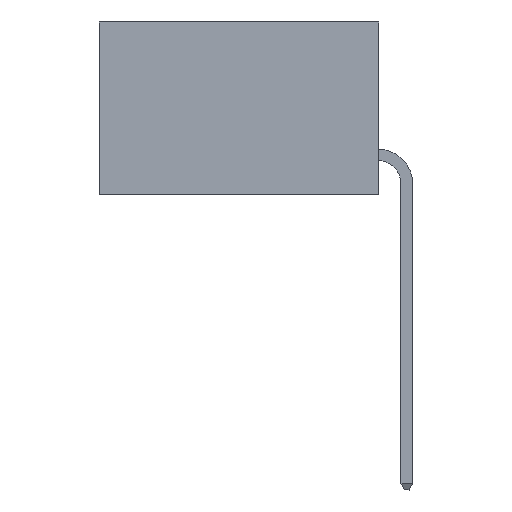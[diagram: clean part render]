
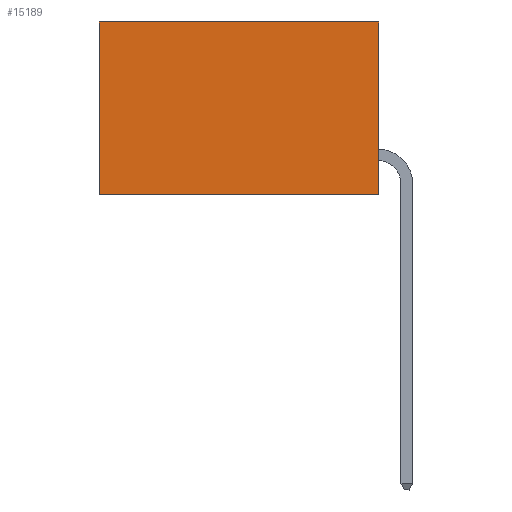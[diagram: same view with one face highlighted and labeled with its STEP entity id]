
A CAD part, left-side view. The second image highlights one B-rep face of the part: STEP entity #15189.
In plain terms, the highlighted planar face has unit normal (-1, 0, 0).
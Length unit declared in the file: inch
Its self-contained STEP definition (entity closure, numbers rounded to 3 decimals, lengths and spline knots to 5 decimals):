
#189 = EDGE_LOOP ( 'NONE', ( #13414, #13663, #11991, #20682 ) ) ;
#394 = CARTESIAN_POINT ( 'NONE',  ( 0.298, 0., 0. ) ) ;
#685 = CARTESIAN_POINT ( 'NONE',  ( 0.298, 0., 0. ) ) ;
#1699 = VERTEX_POINT ( 'NONE', #12876 ) ;
#1809 = DIRECTION ( 'NONE',  ( 0., 1., 0. ) ) ;
#1943 = VECTOR ( 'NONE', #9800, 39.37008 ) ;
#2537 = VECTOR ( 'NONE', #4101, 39.37008 ) ;
#3646 = VERTEX_POINT ( 'NONE', #20419 ) ;
#4101 = DIRECTION ( 'NONE',  ( 0., 0., -1. ) ) ;
#6196 = LINE ( 'NONE', #15282, #1943 ) ;
#7114 = DIRECTION ( 'NONE',  ( 1., 0., 0. ) ) ;
#7199 = EDGE_CURVE ( 'NONE', #17563, #16640, #8212, .T. ) ;
#7425 = DIRECTION ( 'NONE',  ( 0., 0., -1. ) ) ;
#7949 = FACE_OUTER_BOUND ( 'NONE', #189, .T. ) ;
#8212 = LINE ( 'NONE', #20155, #11688 ) ;
#8499 = LINE ( 'NONE', #394, #2537 ) ;
#8904 = CARTESIAN_POINT ( 'NONE',  ( 0.298, 0.6, 0. ) ) ;
#9800 = DIRECTION ( 'NONE',  ( 0., 1., 0. ) ) ;
#10200 = VECTOR ( 'NONE', #7425, 39.37008 ) ;
#11688 = VECTOR ( 'NONE', #1809, 39.37008 ) ;
#11991 = ORIENTED_EDGE ( 'NONE', *, *, #14112, .F. ) ;
#12484 = CARTESIAN_POINT ( 'NONE',  ( 0.298, 0., 0. ) ) ;
#12876 = CARTESIAN_POINT ( 'NONE',  ( 0.298, 0.6, -0.37 ) ) ;
#12893 = CARTESIAN_POINT ( 'NONE',  ( 0.298, 0.6, 0. ) ) ;
#13414 = ORIENTED_EDGE ( 'NONE', *, *, #21513, .T. ) ;
#13663 = ORIENTED_EDGE ( 'NONE', *, *, #21626, .F. ) ;
#14112 = EDGE_CURVE ( 'NONE', #17563, #3646, #8499, .T. ) ;
#14469 = DIRECTION ( 'NONE',  ( 0., 0., -1. ) ) ;
#15189 = ADVANCED_FACE ( 'NONE', ( #7949 ), #23415, .F. ) ;
#15282 = CARTESIAN_POINT ( 'NONE',  ( 0.298, 0., -0.37 ) ) ;
#15662 = LINE ( 'NONE', #12893, #10200 ) ;
#16640 = VERTEX_POINT ( 'NONE', #8904 ) ;
#17563 = VERTEX_POINT ( 'NONE', #685 ) ;
#20155 = CARTESIAN_POINT ( 'NONE',  ( 0.298, 0., 0. ) ) ;
#20419 = CARTESIAN_POINT ( 'NONE',  ( 0.298, 0., -0.37 ) ) ;
#20682 = ORIENTED_EDGE ( 'NONE', *, *, #7199, .T. ) ;
#21513 = EDGE_CURVE ( 'NONE', #16640, #1699, #15662, .T. ) ;
#21626 = EDGE_CURVE ( 'NONE', #3646, #1699, #6196, .T. ) ;
#22619 = AXIS2_PLACEMENT_3D ( 'NONE', #12484, #7114, #14469 ) ;
#23415 = PLANE ( 'NONE',  #22619 ) ;
